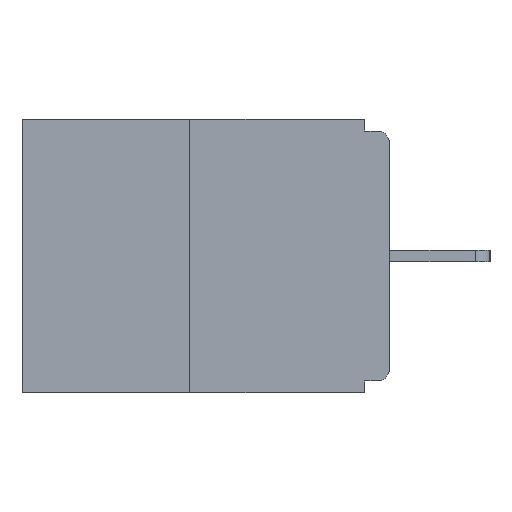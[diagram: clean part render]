
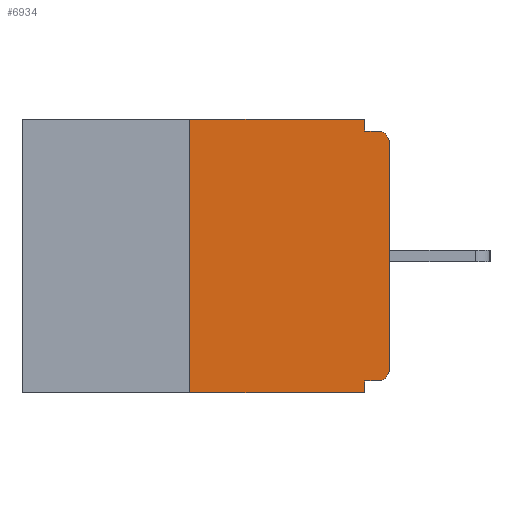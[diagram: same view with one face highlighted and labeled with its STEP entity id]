
A CAD part, left-side view. The second image highlights one B-rep face of the part: STEP entity #6934.
In plain terms, the highlighted planar face has unit normal (-1, 0, 0).
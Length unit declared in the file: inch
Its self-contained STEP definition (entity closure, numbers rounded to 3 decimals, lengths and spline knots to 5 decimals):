
#277 = CARTESIAN_POINT ( 'NONE',  ( 0., 0.031, 0. ) ) ;
#544 = CARTESIAN_POINT ( 'NONE',  ( 0., 0., 0. ) ) ;
#615 = LINE ( 'NONE', #21491, #19277 ) ;
#777 = VECTOR ( 'NONE', #6353, 39.37008 ) ;
#1195 = DIRECTION ( 'NONE',  ( 0., -1., 0. ) ) ;
#1235 = EDGE_CURVE ( 'NONE', #18259, #12777, #3039, .T. ) ;
#1385 = EDGE_CURVE ( 'NONE', #2465, #18259, #5309, .T. ) ;
#1448 = ORIENTED_EDGE ( 'NONE', *, *, #10961, .T. ) ;
#1728 = ORIENTED_EDGE ( 'NONE', *, *, #1385, .F. ) ;
#1735 = VECTOR ( 'NONE', #4047, 39.37008 ) ;
#1746 = EDGE_CURVE ( 'NONE', #12777, #8749, #18596, .T. ) ;
#1880 = CARTESIAN_POINT ( 'NONE',  ( 0., 0.25, 0. ) ) ;
#1887 = DIRECTION ( 'NONE',  ( 1., 0., 0. ) ) ;
#2117 = CARTESIAN_POINT ( 'NONE',  ( 0., 0.031, -0.343 ) ) ;
#2122 = FACE_OUTER_BOUND ( 'NONE', #11800, .T. ) ;
#2465 = VERTEX_POINT ( 'NONE', #4893 ) ;
#2466 = DIRECTION ( 'NONE',  ( 0., 1., 0. ) ) ;
#2940 = CARTESIAN_POINT ( 'NONE',  ( 0., 0.46, -0.343 ) ) ;
#3018 = EDGE_CURVE ( 'NONE', #22385, #20721, #19626, .T. ) ;
#3039 = LINE ( 'NONE', #13349, #777 ) ;
#3609 = CARTESIAN_POINT ( 'NONE',  ( 0., 0.46, 0. ) ) ;
#3693 = DIRECTION ( 'NONE',  ( -1., 0., 0. ) ) ;
#4047 = DIRECTION ( 'NONE',  ( 0., 0., -1. ) ) ;
#4606 = CIRCLE ( 'NONE', #16299, 0.015 ) ;
#4893 = CARTESIAN_POINT ( 'NONE',  ( 0., 0.25, -0.343 ) ) ;
#4910 = DIRECTION ( 'NONE',  ( -1., 0., 0. ) ) ;
#5279 = CIRCLE ( 'NONE', #18082, 0.015 ) ;
#5309 = LINE ( 'NONE', #1880, #11459 ) ;
#5757 = CARTESIAN_POINT ( 'NONE',  ( 0., 0.031, -0.343 ) ) ;
#6117 = VECTOR ( 'NONE', #8282, 39.37008 ) ;
#6353 = DIRECTION ( 'NONE',  ( 0., -1., 0. ) ) ;
#6786 = EDGE_CURVE ( 'NONE', #8749, #17867, #15411, .T. ) ;
#6787 = DIRECTION ( 'NONE',  ( 0., 0., -1. ) ) ;
#6900 = LINE ( 'NONE', #544, #14866 ) ;
#6934 = ADVANCED_FACE ( 'NONE', ( #2122 ), #19301, .F. ) ;
#7279 = EDGE_CURVE ( 'NONE', #12550, #21893, #5279, .T. ) ;
#7438 = ORIENTED_EDGE ( 'NONE', *, *, #1746, .F. ) ;
#7853 = AXIS2_PLACEMENT_3D ( 'NONE', #3609, #1887, #21252 ) ;
#8282 = DIRECTION ( 'NONE',  ( 0., 0., -1. ) ) ;
#8749 = VERTEX_POINT ( 'NONE', #14581 ) ;
#9907 = ORIENTED_EDGE ( 'NONE', *, *, #21435, .T. ) ;
#9927 = LINE ( 'NONE', #2940, #16709 ) ;
#10595 = CARTESIAN_POINT ( 'NONE',  ( 0., 0.015, -0.313 ) ) ;
#10961 = EDGE_CURVE ( 'NONE', #21893, #11968, #6900, .T. ) ;
#11221 = CARTESIAN_POINT ( 'NONE',  ( 0., 0.015, -0.328 ) ) ;
#11459 = VECTOR ( 'NONE', #12320, 39.37008 ) ;
#11515 = ORIENTED_EDGE ( 'NONE', *, *, #6786, .F. ) ;
#11800 = EDGE_LOOP ( 'NONE', ( #21561, #1728, #17606, #21765, #21283, #14514, #1448, #9907, #11515, #7438 ) ) ;
#11968 = VERTEX_POINT ( 'NONE', #18134 ) ;
#12030 = CARTESIAN_POINT ( 'NONE',  ( 0., 0.015, -0.03 ) ) ;
#12320 = DIRECTION ( 'NONE',  ( 0., 0., 1. ) ) ;
#12550 = VERTEX_POINT ( 'NONE', #11221 ) ;
#12777 = VERTEX_POINT ( 'NONE', #277 ) ;
#12883 = EDGE_CURVE ( 'NONE', #12550, #22385, #615, .T. ) ;
#13349 = CARTESIAN_POINT ( 'NONE',  ( 0., 0.46, 0. ) ) ;
#13360 = CARTESIAN_POINT ( 'NONE',  ( 0., 0., -0.015 ) ) ;
#13508 = DIRECTION ( 'NONE',  ( 0., 0., -1. ) ) ;
#13883 = DIRECTION ( 'NONE',  ( 0., 0., 1. ) ) ;
#14514 = ORIENTED_EDGE ( 'NONE', *, *, #7279, .T. ) ;
#14581 = CARTESIAN_POINT ( 'NONE',  ( 0., 0.031, -0.015 ) ) ;
#14866 = VECTOR ( 'NONE', #13883, 39.37008 ) ;
#15068 = DIRECTION ( 'NONE',  ( 0., -1., 0. ) ) ;
#15411 = LINE ( 'NONE', #13360, #16619 ) ;
#16299 = AXIS2_PLACEMENT_3D ( 'NONE', #12030, #4910, #13508 ) ;
#16619 = VECTOR ( 'NONE', #15068, 39.37008 ) ;
#16709 = VECTOR ( 'NONE', #1195, 39.37008 ) ;
#17143 = CARTESIAN_POINT ( 'NONE',  ( 0., 0., -0.313 ) ) ;
#17606 = ORIENTED_EDGE ( 'NONE', *, *, #20615, .T. ) ;
#17867 = VERTEX_POINT ( 'NONE', #22414 ) ;
#18082 = AXIS2_PLACEMENT_3D ( 'NONE', #10595, #3693, #6787 ) ;
#18134 = CARTESIAN_POINT ( 'NONE',  ( 0., 0., -0.03 ) ) ;
#18259 = VERTEX_POINT ( 'NONE', #22427 ) ;
#18596 = LINE ( 'NONE', #21806, #6117 ) ;
#19277 = VECTOR ( 'NONE', #2466, 39.37008 ) ;
#19301 = PLANE ( 'NONE',  #7853 ) ;
#19626 = LINE ( 'NONE', #5757, #1735 ) ;
#20615 = EDGE_CURVE ( 'NONE', #2465, #20721, #9927, .T. ) ;
#20705 = CARTESIAN_POINT ( 'NONE',  ( 0., 0.031, -0.328 ) ) ;
#20721 = VERTEX_POINT ( 'NONE', #2117 ) ;
#21252 = DIRECTION ( 'NONE',  ( 0., 0., -1. ) ) ;
#21283 = ORIENTED_EDGE ( 'NONE', *, *, #12883, .F. ) ;
#21435 = EDGE_CURVE ( 'NONE', #11968, #17867, #4606, .T. ) ;
#21491 = CARTESIAN_POINT ( 'NONE',  ( 0., 0., -0.328 ) ) ;
#21561 = ORIENTED_EDGE ( 'NONE', *, *, #1235, .F. ) ;
#21765 = ORIENTED_EDGE ( 'NONE', *, *, #3018, .F. ) ;
#21806 = CARTESIAN_POINT ( 'NONE',  ( 0., 0.031, 0. ) ) ;
#21893 = VERTEX_POINT ( 'NONE', #17143 ) ;
#22385 = VERTEX_POINT ( 'NONE', #20705 ) ;
#22414 = CARTESIAN_POINT ( 'NONE',  ( 0., 0.015, -0.015 ) ) ;
#22427 = CARTESIAN_POINT ( 'NONE',  ( 0., 0.25, 0. ) ) ;
